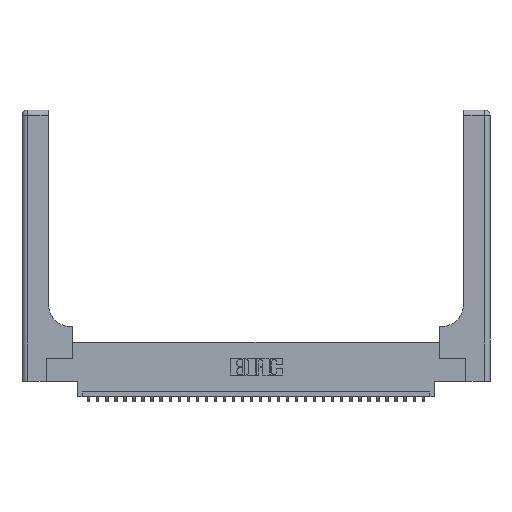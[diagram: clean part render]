
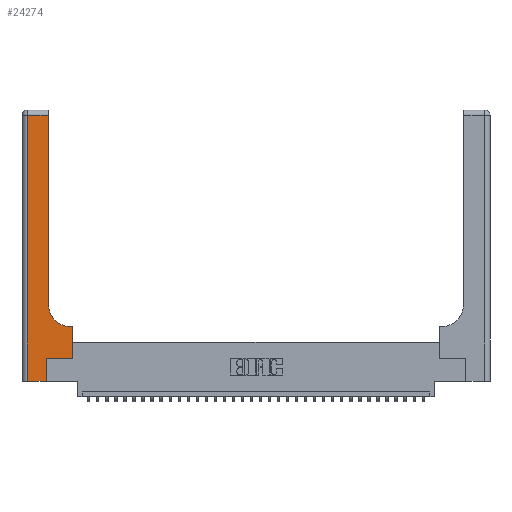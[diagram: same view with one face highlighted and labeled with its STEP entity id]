
A CAD part, top view. The second image highlights one B-rep face of the part: STEP entity #24274.
In plain terms, the highlighted planar face has unit normal (0, 0, 1).
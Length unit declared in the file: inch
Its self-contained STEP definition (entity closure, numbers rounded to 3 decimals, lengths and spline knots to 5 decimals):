
#457 = EDGE_CURVE ( 'NONE', #21851, #3423, #16419, .T. ) ;
#1547 = EDGE_CURVE ( 'NONE', #14691, #6905, #15204, .T. ) ;
#1781 = CARTESIAN_POINT ( 'NONE',  ( 0., 0., 0.37 ) ) ;
#1843 = FACE_OUTER_BOUND ( 'NONE', #20881, .T. ) ;
#1931 = DIRECTION ( 'NONE',  ( 0., 0., -1. ) ) ;
#2000 = CARTESIAN_POINT ( 'NONE',  ( 0.2915, 0.6, 0.37 ) ) ;
#2068 = ORIENTED_EDGE ( 'NONE', *, *, #13935, .T. ) ;
#2253 = CARTESIAN_POINT ( 'NONE',  ( 0.5585, 0.6, 0.37 ) ) ;
#3143 = CARTESIAN_POINT ( 'NONE',  ( 0.269, 0., 0.37 ) ) ;
#3423 = VERTEX_POINT ( 'NONE', #15060 ) ;
#4666 = DIRECTION ( 'NONE',  ( -1., 0., 0. ) ) ;
#4954 = CARTESIAN_POINT ( 'NONE',  ( 0.2915, 2.94, 0.37 ) ) ;
#5395 = LINE ( 'NONE', #23625, #29193 ) ;
#5871 = DIRECTION ( 'NONE',  ( 1., 0., 0. ) ) ;
#6171 = CARTESIAN_POINT ( 'NONE',  ( 0.06, 0., 0.37 ) ) ;
#6422 = VECTOR ( 'NONE', #5871, 39.37008 ) ;
#6655 = LINE ( 'NONE', #1781, #9598 ) ;
#6823 = LINE ( 'NONE', #21883, #6422 ) ;
#6905 = VERTEX_POINT ( 'NONE', #24864 ) ;
#6924 = ORIENTED_EDGE ( 'NONE', *, *, #7103, .T. ) ;
#7103 = EDGE_CURVE ( 'NONE', #26351, #21851, #6655, .T. ) ;
#8960 = LINE ( 'NONE', #26247, #26048 ) ;
#9316 = LINE ( 'NONE', #33390, #32238 ) ;
#9598 = VECTOR ( 'NONE', #31172, 39.37008 ) ;
#9972 = DIRECTION ( 'NONE',  ( -1., 0., 0. ) ) ;
#10011 = EDGE_CURVE ( 'NONE', #3423, #30632, #6823, .T. ) ;
#11620 = DIRECTION ( 'NONE',  ( 0., 1., 0. ) ) ;
#13889 = DIRECTION ( 'NONE',  ( 0., 1., 0. ) ) ;
#13935 = EDGE_CURVE ( 'NONE', #30632, #17355, #9316, .T. ) ;
#14397 = VECTOR ( 'NONE', #4666, 39.37008 ) ;
#14691 = VERTEX_POINT ( 'NONE', #23141 ) ;
#15060 = CARTESIAN_POINT ( 'NONE',  ( 0.269, 0.25, 0.37 ) ) ;
#15204 = CIRCLE ( 'NONE', #26570, 0.25 ) ;
#15606 = DIRECTION ( 'NONE',  ( 1., 0., 0. ) ) ;
#15737 = EDGE_CURVE ( 'NONE', #27226, #26351, #5395, .T. ) ;
#16419 = LINE ( 'NONE', #23673, #25162 ) ;
#17355 = VERTEX_POINT ( 'NONE', #2253 ) ;
#17400 = EDGE_CURVE ( 'NONE', #27327, #27226, #8960, .T. ) ;
#19482 = ORIENTED_EDGE ( 'NONE', *, *, #19768, .T. ) ;
#19768 = EDGE_CURVE ( 'NONE', #6905, #27327, #30753, .T. ) ;
#20243 = DIRECTION ( 'NONE',  ( 0., 0., -1. ) ) ;
#20881 = EDGE_LOOP ( 'NONE', ( #19482, #29097, #22353, #6924, #27859, #33041, #2068, #34322, #26604 ) ) ;
#21851 = VERTEX_POINT ( 'NONE', #3143 ) ;
#21883 = CARTESIAN_POINT ( 'NONE',  ( 0.269, 0.25, 0.37 ) ) ;
#22156 = AXIS2_PLACEMENT_3D ( 'NONE', #25432, #20243, #23599 ) ;
#22353 = ORIENTED_EDGE ( 'NONE', *, *, #15737, .T. ) ;
#22776 = PLANE ( 'NONE',  #22156 ) ;
#23141 = CARTESIAN_POINT ( 'NONE',  ( 0.5415, 0.6, 0.37 ) ) ;
#23599 = DIRECTION ( 'NONE',  ( -1., 0., 0. ) ) ;
#23625 = CARTESIAN_POINT ( 'NONE',  ( 0.06, 3., 0.37 ) ) ;
#23673 = CARTESIAN_POINT ( 'NONE',  ( 0.269, 0., 0.37 ) ) ;
#24106 = VECTOR ( 'NONE', #27562, 39.37008 ) ;
#24274 = ADVANCED_FACE ( 'NONE', ( #1843 ), #22776, .F. ) ;
#24309 = EDGE_CURVE ( 'NONE', #17355, #14691, #27292, .T. ) ;
#24864 = CARTESIAN_POINT ( 'NONE',  ( 0.2915, 0.85, 0.37 ) ) ;
#25162 = VECTOR ( 'NONE', #13889, 39.37008 ) ;
#25432 = CARTESIAN_POINT ( 'NONE',  ( 0., 3., 0.37 ) ) ;
#26048 = VECTOR ( 'NONE', #9972, 39.37008 ) ;
#26247 = CARTESIAN_POINT ( 'NONE',  ( 0., 2.94, 0.37 ) ) ;
#26351 = VERTEX_POINT ( 'NONE', #6171 ) ;
#26570 = AXIS2_PLACEMENT_3D ( 'NONE', #28846, #1931, #15606 ) ;
#26604 = ORIENTED_EDGE ( 'NONE', *, *, #1547, .T. ) ;
#27226 = VERTEX_POINT ( 'NONE', #29201 ) ;
#27292 = LINE ( 'NONE', #2000, #14397 ) ;
#27327 = VERTEX_POINT ( 'NONE', #4954 ) ;
#27562 = DIRECTION ( 'NONE',  ( 0., 1., 0. ) ) ;
#27859 = ORIENTED_EDGE ( 'NONE', *, *, #457, .T. ) ;
#28846 = CARTESIAN_POINT ( 'NONE',  ( 0.5415, 0.85, 0.37 ) ) ;
#29097 = ORIENTED_EDGE ( 'NONE', *, *, #17400, .T. ) ;
#29193 = VECTOR ( 'NONE', #29675, 39.37008 ) ;
#29201 = CARTESIAN_POINT ( 'NONE',  ( 0.06, 2.94, 0.37 ) ) ;
#29675 = DIRECTION ( 'NONE',  ( 0., -1., 0. ) ) ;
#30632 = VERTEX_POINT ( 'NONE', #30802 ) ;
#30753 = LINE ( 'NONE', #32818, #24106 ) ;
#30802 = CARTESIAN_POINT ( 'NONE',  ( 0.5585, 0.25, 0.37 ) ) ;
#31172 = DIRECTION ( 'NONE',  ( 1., 0., 0. ) ) ;
#32238 = VECTOR ( 'NONE', #11620, 39.37008 ) ;
#32818 = CARTESIAN_POINT ( 'NONE',  ( 0.2915, 3., 0.37 ) ) ;
#33041 = ORIENTED_EDGE ( 'NONE', *, *, #10011, .T. ) ;
#33390 = CARTESIAN_POINT ( 'NONE',  ( 0.5585, 0.25, 0.37 ) ) ;
#34322 = ORIENTED_EDGE ( 'NONE', *, *, #24309, .T. ) ;
